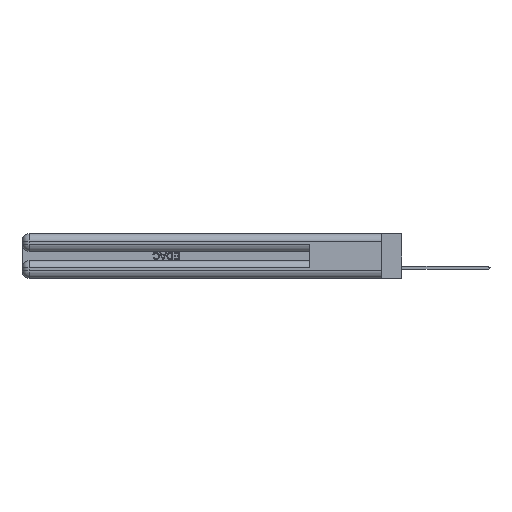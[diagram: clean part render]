
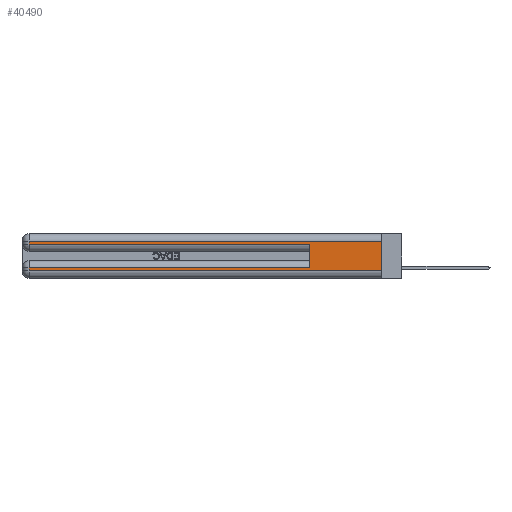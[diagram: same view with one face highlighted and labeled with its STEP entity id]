
A CAD part, left-side view. The second image highlights one B-rep face of the part: STEP entity #40490.
In plain terms, the highlighted planar face has unit normal (-1, 0, 0).
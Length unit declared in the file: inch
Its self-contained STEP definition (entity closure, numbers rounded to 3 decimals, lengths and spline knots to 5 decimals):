
#512 = VECTOR ( 'NONE', #2805, 39.37008 ) ;
#570 = VECTOR ( 'NONE', #5676, 39.37008 ) ;
#1174 = VECTOR ( 'NONE', #7162, 39.37008 ) ;
#1210 = VERTEX_POINT ( 'NONE', #17568 ) ;
#1502 = LINE ( 'NONE', #33913, #512 ) ;
#1846 = CARTESIAN_POINT ( 'NONE',  ( 0., 0., 0.31 ) ) ;
#2167 = DIRECTION ( 'NONE',  ( 0., 0., -1. ) ) ;
#2805 = DIRECTION ( 'NONE',  ( 0., -1., 0. ) ) ;
#3175 = EDGE_CURVE ( 'NONE', #10883, #31461, #37553, .T. ) ;
#4330 = LINE ( 'NONE', #37011, #28338 ) ;
#5336 = CARTESIAN_POINT ( 'NONE',  ( 0., 0.6, 0.285 ) ) ;
#5529 = EDGE_CURVE ( 'NONE', #20209, #1210, #25618, .T. ) ;
#5676 = DIRECTION ( 'NONE',  ( 0., 1., 0. ) ) ;
#6562 = VERTEX_POINT ( 'NONE', #25885 ) ;
#6601 = CARTESIAN_POINT ( 'NONE',  ( 0., 0.6, 0.085 ) ) ;
#7077 = VECTOR ( 'NONE', #36415, 39.37008 ) ;
#7162 = DIRECTION ( 'NONE',  ( 0., 0., -1. ) ) ;
#7529 = AXIS2_PLACEMENT_3D ( 'NONE', #24366, #30674, #36705 ) ;
#10012 = ORIENTED_EDGE ( 'NONE', *, *, #11097, .T. ) ;
#10856 = EDGE_CURVE ( 'NONE', #10883, #12612, #33544, .T. ) ;
#10883 = VERTEX_POINT ( 'NONE', #21238 ) ;
#11025 = CARTESIAN_POINT ( 'NONE',  ( 0., 0., 0.06 ) ) ;
#11037 = ORIENTED_EDGE ( 'NONE', *, *, #37740, .T. ) ;
#11097 = EDGE_CURVE ( 'NONE', #12612, #23039, #16377, .T. ) ;
#11876 = CARTESIAN_POINT ( 'NONE',  ( 0., 0., 0.06 ) ) ;
#12612 = VERTEX_POINT ( 'NONE', #36948 ) ;
#13291 = EDGE_CURVE ( 'NONE', #23039, #29365, #1502, .T. ) ;
#13477 = ORIENTED_EDGE ( 'NONE', *, *, #28465, .T. ) ;
#14674 = VECTOR ( 'NONE', #2167, 39.37008 ) ;
#15004 = EDGE_CURVE ( 'NONE', #20209, #29365, #4330, .T. ) ;
#16112 = ORIENTED_EDGE ( 'NONE', *, *, #13291, .T. ) ;
#16377 = LINE ( 'NONE', #38948, #1174 ) ;
#16820 = ORIENTED_EDGE ( 'NONE', *, *, #5529, .T. ) ;
#17568 = CARTESIAN_POINT ( 'NONE',  ( 0., 2.94, 0.085 ) ) ;
#20209 = VERTEX_POINT ( 'NONE', #6601 ) ;
#20840 = CARTESIAN_POINT ( 'NONE',  ( 0., 2.94, 0.37 ) ) ;
#21157 = CARTESIAN_POINT ( 'NONE',  ( 0., 0., 0.085 ) ) ;
#21238 = CARTESIAN_POINT ( 'NONE',  ( 0., 0., 0.31 ) ) ;
#22851 = VECTOR ( 'NONE', #37040, 39.37008 ) ;
#23039 = VERTEX_POINT ( 'NONE', #32506 ) ;
#24366 = CARTESIAN_POINT ( 'NONE',  ( 0., 0., 0.37 ) ) ;
#25618 = LINE ( 'NONE', #21157, #570 ) ;
#25885 = CARTESIAN_POINT ( 'NONE',  ( 0., 2.94, 0.06 ) ) ;
#27309 = EDGE_LOOP ( 'NONE', ( #30728, #35963, #10012, #16112, #35966, #16820, #11037, #13477 ) ) ;
#28338 = VECTOR ( 'NONE', #30967, 39.37008 ) ;
#28389 = VECTOR ( 'NONE', #38964, 39.37008 ) ;
#28465 = EDGE_CURVE ( 'NONE', #6562, #31461, #36798, .T. ) ;
#29365 = VERTEX_POINT ( 'NONE', #5336 ) ;
#30599 = FACE_OUTER_BOUND ( 'NONE', #27309, .T. ) ;
#30674 = DIRECTION ( 'NONE',  ( 1., 0., 0. ) ) ;
#30728 = ORIENTED_EDGE ( 'NONE', *, *, #3175, .F. ) ;
#30967 = DIRECTION ( 'NONE',  ( 0., 0., 1. ) ) ;
#31129 = CARTESIAN_POINT ( 'NONE',  ( 0., 0., 0.37 ) ) ;
#31325 = LINE ( 'NONE', #20840, #14674 ) ;
#31461 = VERTEX_POINT ( 'NONE', #11876 ) ;
#32506 = CARTESIAN_POINT ( 'NONE',  ( 0., 2.94, 0.285 ) ) ;
#33247 = PLANE ( 'NONE',  #7529 ) ;
#33544 = LINE ( 'NONE', #1846, #7077 ) ;
#33913 = CARTESIAN_POINT ( 'NONE',  ( 0., 0., 0.285 ) ) ;
#35963 = ORIENTED_EDGE ( 'NONE', *, *, #10856, .T. ) ;
#35966 = ORIENTED_EDGE ( 'NONE', *, *, #15004, .F. ) ;
#36415 = DIRECTION ( 'NONE',  ( 0., 1., 0. ) ) ;
#36705 = DIRECTION ( 'NONE',  ( 0., 0., -1. ) ) ;
#36798 = LINE ( 'NONE', #11025, #28389 ) ;
#36948 = CARTESIAN_POINT ( 'NONE',  ( 0., 2.94, 0.31 ) ) ;
#37011 = CARTESIAN_POINT ( 'NONE',  ( 0., 0.6, 0.145 ) ) ;
#37040 = DIRECTION ( 'NONE',  ( 0., 0., -1. ) ) ;
#37553 = LINE ( 'NONE', #31129, #22851 ) ;
#37740 = EDGE_CURVE ( 'NONE', #1210, #6562, #31325, .T. ) ;
#38948 = CARTESIAN_POINT ( 'NONE',  ( 0., 2.94, 0.37 ) ) ;
#38964 = DIRECTION ( 'NONE',  ( 0., -1., 0. ) ) ;
#40490 = ADVANCED_FACE ( 'NONE', ( #30599 ), #33247, .F. ) ;
